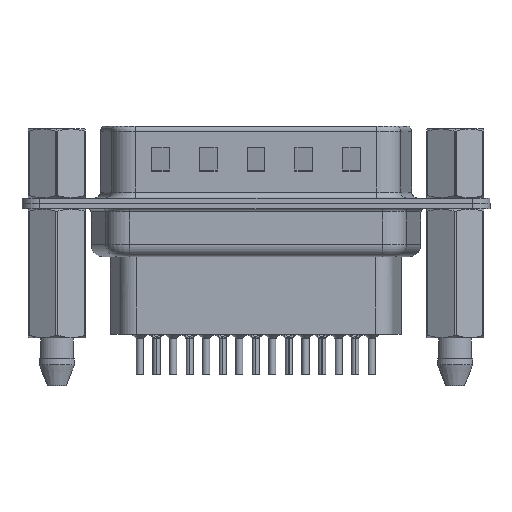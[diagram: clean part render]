
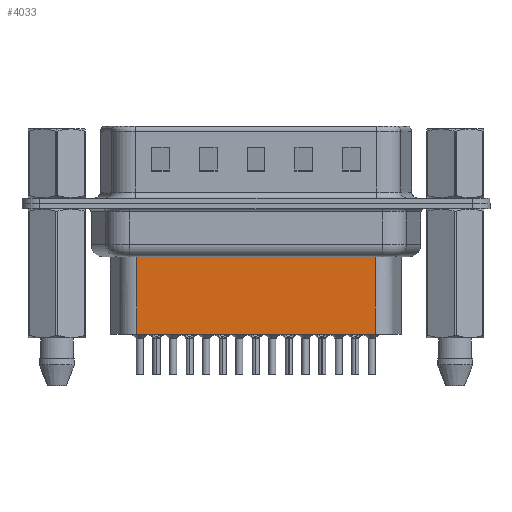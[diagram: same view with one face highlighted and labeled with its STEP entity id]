
A CAD part, front view. The second image highlights one B-rep face of the part: STEP entity #4033.
In plain terms, the highlighted planar face has unit normal (0, -1, 0).
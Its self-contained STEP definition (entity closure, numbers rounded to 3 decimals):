
#2094 = VERTEX_POINT ( 'NONE', #21706 ) ;
#2657 = LINE ( 'NONE', #8999, #28243 ) ;
#3687 = CARTESIAN_POINT ( 'NONE',  ( 6.434, -3.5, -4.097 ) ) ;
#3775 = VERTEX_POINT ( 'NONE', #18799 ) ;
#4033 = ADVANCED_FACE ( 'NONE', ( #4158 ), #9122, .T. ) ;
#4158 = FACE_OUTER_BOUND ( 'NONE', #19280, .T. ) ;
#4840 = ORIENTED_EDGE ( 'NONE', *, *, #20506, .F. ) ;
#6265 = DIRECTION ( 'NONE',  ( 0., -1., 0. ) ) ;
#6708 = DIRECTION ( 'NONE',  ( 1., 0., 0. ) ) ;
#7128 = EDGE_CURVE ( 'NONE', #17875, #2094, #22305, .T. ) ;
#8981 = ORIENTED_EDGE ( 'NONE', *, *, #21848, .T. ) ;
#8999 = CARTESIAN_POINT ( 'NONE',  ( 26.619, -3.5, -3.1 ) ) ;
#9122 = PLANE ( 'NONE',  #22317 ) ;
#13190 = CARTESIAN_POINT ( 'NONE',  ( 26.619, -3.5, -4.097 ) ) ;
#13240 = CARTESIAN_POINT ( 'NONE',  ( 6.681, -3.5, -10.95 ) ) ;
#16151 = CARTESIAN_POINT ( 'NONE',  ( 6.681, -3.5, -3.1 ) ) ;
#17826 = VECTOR ( 'NONE', #18407, 1000. ) ;
#17875 = VERTEX_POINT ( 'NONE', #21734 ) ;
#18081 = ORIENTED_EDGE ( 'NONE', *, *, #26289, .T. ) ;
#18407 = DIRECTION ( 'NONE',  ( 0., 0., -1. ) ) ;
#18697 = LINE ( 'NONE', #16151, #17826 ) ;
#18799 = CARTESIAN_POINT ( 'NONE',  ( 6.681, -3.5, -4.097 ) ) ;
#18929 = ORIENTED_EDGE ( 'NONE', *, *, #7128, .F. ) ;
#19280 = EDGE_LOOP ( 'NONE', ( #4840, #18081, #8981, #18929 ) ) ;
#19525 = VECTOR ( 'NONE', #19880, 1000. ) ;
#19880 = DIRECTION ( 'NONE',  ( -1., 0., 0. ) ) ;
#20337 = DIRECTION ( 'NONE',  ( 0., 0., -1. ) ) ;
#20355 = VECTOR ( 'NONE', #24203, 1000. ) ;
#20454 = CARTESIAN_POINT ( 'NONE',  ( 6.681, -3.5, -3.1 ) ) ;
#20506 = EDGE_CURVE ( 'NONE', #27797, #17875, #2657, .T. ) ;
#21706 = CARTESIAN_POINT ( 'NONE',  ( 6.681, -3.5, -10.95 ) ) ;
#21734 = CARTESIAN_POINT ( 'NONE',  ( 26.619, -3.5, -10.95 ) ) ;
#21789 = LINE ( 'NONE', #3687, #20355 ) ;
#21848 = EDGE_CURVE ( 'NONE', #3775, #2094, #18697, .T. ) ;
#22305 = LINE ( 'NONE', #13240, #19525 ) ;
#22317 = AXIS2_PLACEMENT_3D ( 'NONE', #20454, #6265, #6708 ) ;
#24203 = DIRECTION ( 'NONE',  ( -1., 0., 0. ) ) ;
#26289 = EDGE_CURVE ( 'NONE', #27797, #3775, #21789, .T. ) ;
#27797 = VERTEX_POINT ( 'NONE', #13190 ) ;
#28243 = VECTOR ( 'NONE', #20337, 1000. ) ;
